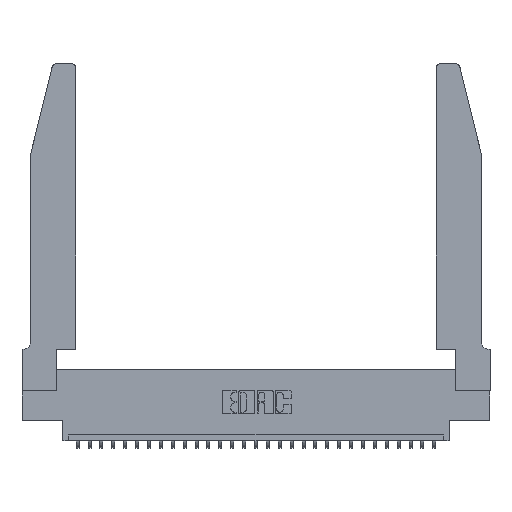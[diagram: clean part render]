
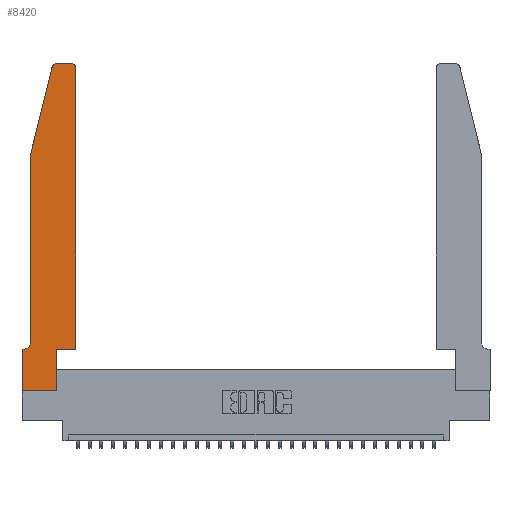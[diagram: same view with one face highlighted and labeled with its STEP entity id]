
A CAD part, top view. The second image highlights one B-rep face of the part: STEP entity #8420.
In plain terms, the highlighted planar face has unit normal (0, 0, 1).
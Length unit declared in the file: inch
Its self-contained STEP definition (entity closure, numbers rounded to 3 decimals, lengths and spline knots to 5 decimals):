
#364 = VECTOR ( 'NONE', #22970, 39.37008 ) ;
#795 = CARTESIAN_POINT ( 'NONE',  ( 0.25487, 2.72718, 0.37 ) ) ;
#1151 = PLANE ( 'NONE',  #5192 ) ;
#1339 = ORIENTED_EDGE ( 'NONE', *, *, #13551, .T. ) ;
#1530 = CIRCLE ( 'NONE', #22744, 0.03 ) ;
#1655 = DIRECTION ( 'NONE',  ( 0., -1., 0. ) ) ;
#1657 = VERTEX_POINT ( 'NONE', #6638 ) ;
#1666 = LINE ( 'NONE', #28636, #15346 ) ;
#1747 = DIRECTION ( 'NONE',  ( 0., -1., 0. ) ) ;
#2192 = CARTESIAN_POINT ( 'NONE',  ( 0.4505, 0.35, 0.37 ) ) ;
#2261 = FACE_OUTER_BOUND ( 'NONE', #5418, .T. ) ;
#2759 = AXIS2_PLACEMENT_3D ( 'NONE', #20200, #6418, #15657 ) ;
#2944 = EDGE_CURVE ( 'NONE', #18057, #19702, #1530, .T. ) ;
#3384 = EDGE_CURVE ( 'NONE', #3511, #19804, #13016, .T. ) ;
#3511 = VERTEX_POINT ( 'NONE', #17161 ) ;
#3528 = ORIENTED_EDGE ( 'NONE', *, *, #2944, .T. ) ;
#4410 = VECTOR ( 'NONE', #15550, 39.37008 ) ;
#4461 = ORIENTED_EDGE ( 'NONE', *, *, #12275, .T. ) ;
#4835 = CARTESIAN_POINT ( 'NONE',  ( 0.4205, 2.75, 0.37 ) ) ;
#5192 = AXIS2_PLACEMENT_3D ( 'NONE', #17236, #19549, #10361 ) ;
#5418 = EDGE_LOOP ( 'NONE', ( #5731, #3528, #12700, #25691, #17383, #1339, #4461, #9774, #23518, #19464, #21512, #19263 ) ) ;
#5431 = AXIS2_PLACEMENT_3D ( 'NONE', #9896, #7601, #18979 ) ;
#5731 = ORIENTED_EDGE ( 'NONE', *, *, #15810, .T. ) ;
#6191 = VECTOR ( 'NONE', #24183, 39.37008 ) ;
#6288 = DIRECTION ( 'NONE',  ( 0., 1., 0. ) ) ;
#6418 = DIRECTION ( 'NONE',  ( 0., 0., 1. ) ) ;
#6484 = LINE ( 'NONE', #2192, #364 ) ;
#6638 = CARTESIAN_POINT ( 'NONE',  ( 0.0755, 2., 0.37 ) ) ;
#6812 = CIRCLE ( 'NONE', #2759, 0.03 ) ;
#6909 = LINE ( 'NONE', #28604, #4410 ) ;
#6929 = CARTESIAN_POINT ( 'NONE',  ( 0., 0.35, 0.37 ) ) ;
#7480 = VERTEX_POINT ( 'NONE', #9317 ) ;
#7601 = DIRECTION ( 'NONE',  ( 0., 0., -1. ) ) ;
#8036 = DIRECTION ( 'NONE',  ( 1., 0., 0. ) ) ;
#8420 = ADVANCED_FACE ( 'NONE', ( #2261 ), #1151, .T. ) ;
#8475 = VECTOR ( 'NONE', #6288, 39.37008 ) ;
#8846 = VECTOR ( 'NONE', #1655, 39.37008 ) ;
#8942 = CARTESIAN_POINT ( 'NONE',  ( 0.284, 2.75, 0.37 ) ) ;
#9317 = CARTESIAN_POINT ( 'NONE',  ( 0., 0., 0.37 ) ) ;
#9774 = ORIENTED_EDGE ( 'NONE', *, *, #28585, .T. ) ;
#9896 = CARTESIAN_POINT ( 'NONE',  ( 0.0055, 0.42, 0.37 ) ) ;
#10236 = DIRECTION ( 'NONE',  ( 1., 0., 0. ) ) ;
#10279 = LINE ( 'NONE', #17557, #8846 ) ;
#10361 = DIRECTION ( 'NONE',  ( 1., 0., 0. ) ) ;
#10579 = EDGE_CURVE ( 'NONE', #21191, #27316, #6484, .T. ) ;
#10908 = EDGE_CURVE ( 'NONE', #29222, #26060, #6812, .T. ) ;
#11030 = LINE ( 'NONE', #18094, #29387 ) ;
#12275 = EDGE_CURVE ( 'NONE', #24840, #7480, #24407, .T. ) ;
#12609 = CARTESIAN_POINT ( 'NONE',  ( 0., 0., 0.37 ) ) ;
#12700 = ORIENTED_EDGE ( 'NONE', *, *, #25232, .T. ) ;
#13016 = CIRCLE ( 'NONE', #5431, 0.07 ) ;
#13551 = EDGE_CURVE ( 'NONE', #19804, #24840, #16778, .T. ) ;
#14169 = CARTESIAN_POINT ( 'NONE',  ( 0.4505, 0.35, 0.37 ) ) ;
#14479 = LINE ( 'NONE', #15365, #6191 ) ;
#14620 = LINE ( 'NONE', #17858, #8475 ) ;
#15006 = CARTESIAN_POINT ( 'NONE',  ( 0.0755, 0.35, 0.37 ) ) ;
#15346 = VECTOR ( 'NONE', #10236, 39.37008 ) ;
#15365 = CARTESIAN_POINT ( 'NONE',  ( 0.0755, 2., 0.37 ) ) ;
#15425 = VECTOR ( 'NONE', #1747, 39.37008 ) ;
#15550 = DIRECTION ( 'NONE',  ( -1., 0., 0. ) ) ;
#15657 = DIRECTION ( 'NONE',  ( 1., 0., 0. ) ) ;
#15810 = EDGE_CURVE ( 'NONE', #26060, #18057, #6909, .T. ) ;
#16778 = LINE ( 'NONE', #15006, #26819 ) ;
#17161 = CARTESIAN_POINT ( 'NONE',  ( 0.0755, 0.42, 0.37 ) ) ;
#17236 = CARTESIAN_POINT ( 'NONE',  ( 0., 0.35, 0.37 ) ) ;
#17383 = ORIENTED_EDGE ( 'NONE', *, *, #3384, .T. ) ;
#17497 = CARTESIAN_POINT ( 'NONE',  ( 0.2865, 0.35, 0.37 ) ) ;
#17557 = CARTESIAN_POINT ( 'NONE',  ( 0.0755, 2., 0.37 ) ) ;
#17858 = CARTESIAN_POINT ( 'NONE',  ( 0.4505, 0.35, 0.37 ) ) ;
#18057 = VERTEX_POINT ( 'NONE', #8942 ) ;
#18094 = CARTESIAN_POINT ( 'NONE',  ( 0.2865, 0.35, 0.37 ) ) ;
#18979 = DIRECTION ( 'NONE',  ( -1., 0., 0. ) ) ;
#19111 = CARTESIAN_POINT ( 'NONE',  ( 0.4505, 2.72, 0.37 ) ) ;
#19263 = ORIENTED_EDGE ( 'NONE', *, *, #10908, .T. ) ;
#19464 = ORIENTED_EDGE ( 'NONE', *, *, #10579, .T. ) ;
#19549 = DIRECTION ( 'NONE',  ( 0., 0., 1. ) ) ;
#19702 = VERTEX_POINT ( 'NONE', #795 ) ;
#19804 = VERTEX_POINT ( 'NONE', #24180 ) ;
#20195 = DIRECTION ( 'NONE',  ( 0., 1., 0. ) ) ;
#20200 = CARTESIAN_POINT ( 'NONE',  ( 0.4205, 2.72, 0.37 ) ) ;
#21191 = VERTEX_POINT ( 'NONE', #17497 ) ;
#21512 = ORIENTED_EDGE ( 'NONE', *, *, #23993, .T. ) ;
#22026 = DIRECTION ( 'NONE',  ( 0., 0., 1. ) ) ;
#22744 = AXIS2_PLACEMENT_3D ( 'NONE', #24208, #22026, #8036 ) ;
#22970 = DIRECTION ( 'NONE',  ( 1., 0., 0. ) ) ;
#23518 = ORIENTED_EDGE ( 'NONE', *, *, #27487, .T. ) ;
#23993 = EDGE_CURVE ( 'NONE', #27316, #29222, #14620, .T. ) ;
#24124 = DIRECTION ( 'NONE',  ( -1., 0., 0. ) ) ;
#24180 = CARTESIAN_POINT ( 'NONE',  ( 0.0055, 0.35, 0.37 ) ) ;
#24183 = DIRECTION ( 'NONE',  ( -0.239, -0.971, 0. ) ) ;
#24208 = CARTESIAN_POINT ( 'NONE',  ( 0.284, 2.72, 0.37 ) ) ;
#24407 = LINE ( 'NONE', #12609, #15425 ) ;
#24840 = VERTEX_POINT ( 'NONE', #6929 ) ;
#25232 = EDGE_CURVE ( 'NONE', #19702, #1657, #14479, .T. ) ;
#25691 = ORIENTED_EDGE ( 'NONE', *, *, #28064, .T. ) ;
#26060 = VERTEX_POINT ( 'NONE', #4835 ) ;
#26410 = CARTESIAN_POINT ( 'NONE',  ( 0.2865, 0., 0.37 ) ) ;
#26819 = VECTOR ( 'NONE', #24124, 39.37008 ) ;
#27316 = VERTEX_POINT ( 'NONE', #14169 ) ;
#27487 = EDGE_CURVE ( 'NONE', #29318, #21191, #11030, .T. ) ;
#28064 = EDGE_CURVE ( 'NONE', #1657, #3511, #10279, .T. ) ;
#28585 = EDGE_CURVE ( 'NONE', #7480, #29318, #1666, .T. ) ;
#28604 = CARTESIAN_POINT ( 'NONE',  ( 0.2605, 2.75, 0.37 ) ) ;
#28636 = CARTESIAN_POINT ( 'NONE',  ( 0., 0., 0.37 ) ) ;
#29222 = VERTEX_POINT ( 'NONE', #19111 ) ;
#29318 = VERTEX_POINT ( 'NONE', #26410 ) ;
#29387 = VECTOR ( 'NONE', #20195, 39.37008 ) ;
